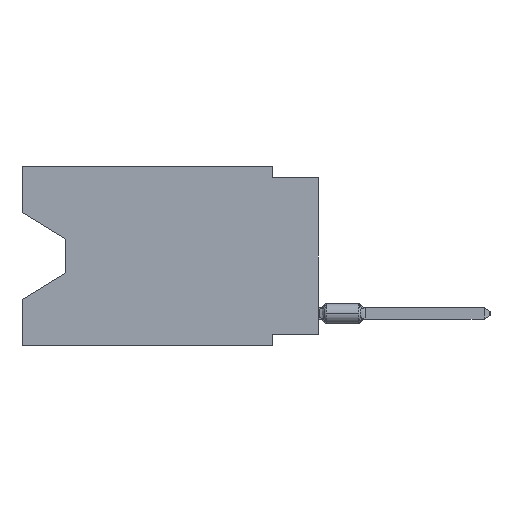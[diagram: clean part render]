
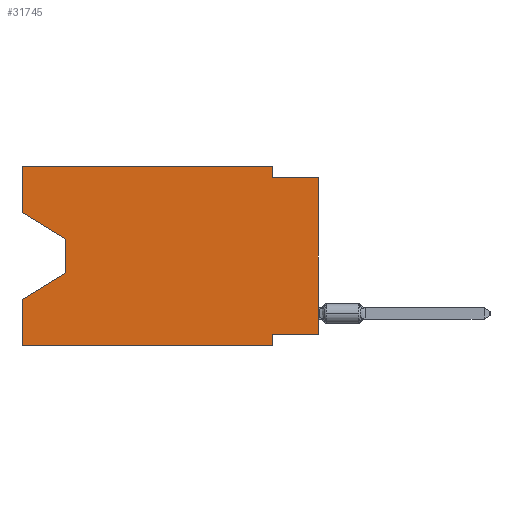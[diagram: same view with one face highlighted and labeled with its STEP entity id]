
A CAD part, left-side view. The second image highlights one B-rep face of the part: STEP entity #31745.
In plain terms, the highlighted planar face has unit normal (-1, 0, 0).
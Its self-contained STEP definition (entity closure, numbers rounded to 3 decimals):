
#317 = CARTESIAN_POINT ( 'NONE',  ( 0., 2.54, 0. ) ) ;
#794 = CARTESIAN_POINT ( 'NONE',  ( 0., 16.383, -7.36 ) ) ;
#2900 = EDGE_CURVE ( 'NONE', #40941, #24590, #13201, .T. ) ;
#3535 = CARTESIAN_POINT ( 'NONE',  ( 0., 2.54, -9.271 ) ) ;
#3606 = ORIENTED_EDGE ( 'NONE', *, *, #37681, .F. ) ;
#3652 = EDGE_CURVE ( 'NONE', #67904, #61742, #54714, .T. ) ;
#5133 = EDGE_CURVE ( 'NONE', #24590, #61742, #12142, .T. ) ;
#5158 = DIRECTION ( 'NONE',  ( 0., 0., -1. ) ) ;
#6600 = CARTESIAN_POINT ( 'NONE',  ( 0., 0., -0.635 ) ) ;
#6945 = ORIENTED_EDGE ( 'NONE', *, *, #54224, .T. ) ;
#7548 = EDGE_LOOP ( 'NONE', ( #6945, #16063, #22854, #64607, #65771, #75568, #11442, #66513, #3606, #39888, #7918, #61162 ) ) ;
#7918 = ORIENTED_EDGE ( 'NONE', *, *, #39443, .F. ) ;
#9223 = VECTOR ( 'NONE', #51706, 1000. ) ;
#10031 = EDGE_CURVE ( 'NONE', #40941, #60009, #31237, .T. ) ;
#11442 = ORIENTED_EDGE ( 'NONE', *, *, #2900, .F. ) ;
#12142 = LINE ( 'NONE', #12539, #59443 ) ;
#12539 = CARTESIAN_POINT ( 'NONE',  ( 0., 2.54, -9.906 ) ) ;
#12834 = EDGE_CURVE ( 'NONE', #67904, #27553, #40180, .T. ) ;
#13201 = LINE ( 'NONE', #73560, #40189 ) ;
#13399 = CARTESIAN_POINT ( 'NONE',  ( 0., 16.383, -9.906 ) ) ;
#16031 = VERTEX_POINT ( 'NONE', #59079 ) ;
#16063 = ORIENTED_EDGE ( 'NONE', *, *, #67375, .T. ) ;
#18263 = FACE_OUTER_BOUND ( 'NONE', #7548, .T. ) ;
#19189 = LINE ( 'NONE', #44994, #19703 ) ;
#19703 = VECTOR ( 'NONE', #19977, 1000. ) ;
#19977 = DIRECTION ( 'NONE',  ( 0., 0., -1. ) ) ;
#22854 = ORIENTED_EDGE ( 'NONE', *, *, #23159, .T. ) ;
#23034 = CARTESIAN_POINT ( 'NONE',  ( 0., 13.97, -5.893 ) ) ;
#23159 = EDGE_CURVE ( 'NONE', #16031, #27553, #48436, .T. ) ;
#24590 = VERTEX_POINT ( 'NONE', #3535 ) ;
#24606 = DIRECTION ( 'NONE',  ( 1., 0., 0. ) ) ;
#25218 = DIRECTION ( 'NONE',  ( 0., 0., -1. ) ) ;
#25721 = VERTEX_POINT ( 'NONE', #63692 ) ;
#27425 = CARTESIAN_POINT ( 'NONE',  ( 0., 0., -9.271 ) ) ;
#27553 = VERTEX_POINT ( 'NONE', #794 ) ;
#28257 = DIRECTION ( 'NONE',  ( 0., 0., 1. ) ) ;
#29636 = LINE ( 'NONE', #30027, #42923 ) ;
#30027 = CARTESIAN_POINT ( 'NONE',  ( 0., 16.383, -2.546 ) ) ;
#30146 = VECTOR ( 'NONE', #28257, 1000. ) ;
#30824 = DIRECTION ( 'NONE',  ( 0., -1., 0. ) ) ;
#31237 = LINE ( 'NONE', #37596, #67380 ) ;
#31328 = VECTOR ( 'NONE', #30824, 1000. ) ;
#31745 = ADVANCED_FACE ( 'NONE', ( #18263 ), #48042, .F. ) ;
#32896 = AXIS2_PLACEMENT_3D ( 'NONE', #42490, #24606, #5158 ) ;
#34213 = LINE ( 'NONE', #65194, #30146 ) ;
#37596 = CARTESIAN_POINT ( 'NONE',  ( 0., 0., 0. ) ) ;
#37681 = EDGE_CURVE ( 'NONE', #68597, #60009, #49102, .T. ) ;
#38248 = CARTESIAN_POINT ( 'NONE',  ( 0., 2.54, -0.635 ) ) ;
#38661 = CARTESIAN_POINT ( 'NONE',  ( 0., 16.383, 0. ) ) ;
#38982 = VECTOR ( 'NONE', #43185, 1000. ) ;
#39041 = LINE ( 'NONE', #38661, #71755 ) ;
#39443 = EDGE_CURVE ( 'NONE', #25721, #65677, #39041, .T. ) ;
#39522 = VERTEX_POINT ( 'NONE', #64465 ) ;
#39888 = ORIENTED_EDGE ( 'NONE', *, *, #53935, .F. ) ;
#40180 = LINE ( 'NONE', #64412, #9223 ) ;
#40189 = VECTOR ( 'NONE', #61636, 1000. ) ;
#40941 = VERTEX_POINT ( 'NONE', #27425 ) ;
#41727 = VECTOR ( 'NONE', #54413, 1000. ) ;
#42490 = CARTESIAN_POINT ( 'NONE',  ( 0., 16.383, 0. ) ) ;
#42826 = DIRECTION ( 'NONE',  ( 0., 0., -1. ) ) ;
#42923 = VECTOR ( 'NONE', #47514, 1000. ) ;
#43185 = DIRECTION ( 'NONE',  ( 0., -1., 0. ) ) ;
#43878 = CARTESIAN_POINT ( 'NONE',  ( 0., 16.383, -9.906 ) ) ;
#44994 = CARTESIAN_POINT ( 'NONE',  ( 0., 13.97, -4.013 ) ) ;
#47302 = CARTESIAN_POINT ( 'NONE',  ( 0., 2.54, -9.906 ) ) ;
#47514 = DIRECTION ( 'NONE',  ( 0., -0.855, -0.519 ) ) ;
#48042 = PLANE ( 'NONE',  #32896 ) ;
#48436 = LINE ( 'NONE', #23034, #41727 ) ;
#49102 = LINE ( 'NONE', #6600, #31328 ) ;
#51706 = DIRECTION ( 'NONE',  ( 0., 0., 1. ) ) ;
#53387 = EDGE_CURVE ( 'NONE', #39522, #25721, #34213, .T. ) ;
#53935 = EDGE_CURVE ( 'NONE', #65677, #68597, #54742, .T. ) ;
#54224 = EDGE_CURVE ( 'NONE', #39522, #59532, #29636, .T. ) ;
#54413 = DIRECTION ( 'NONE',  ( 0., 0.855, -0.519 ) ) ;
#54714 = LINE ( 'NONE', #13399, #38982 ) ;
#54742 = LINE ( 'NONE', #317, #74623 ) ;
#59079 = CARTESIAN_POINT ( 'NONE',  ( 0., 13.97, -5.893 ) ) ;
#59443 = VECTOR ( 'NONE', #25218, 1000. ) ;
#59532 = VERTEX_POINT ( 'NONE', #74659 ) ;
#59787 = CARTESIAN_POINT ( 'NONE',  ( 0., 0., -0.635 ) ) ;
#59808 = CARTESIAN_POINT ( 'NONE',  ( 0., 2.54, 0. ) ) ;
#60009 = VERTEX_POINT ( 'NONE', #59787 ) ;
#60640 = DIRECTION ( 'NONE',  ( 0., 0., 1. ) ) ;
#61162 = ORIENTED_EDGE ( 'NONE', *, *, #53387, .F. ) ;
#61636 = DIRECTION ( 'NONE',  ( 0., 1., 0. ) ) ;
#61742 = VERTEX_POINT ( 'NONE', #47302 ) ;
#63683 = DIRECTION ( 'NONE',  ( 0., -1., 0. ) ) ;
#63692 = CARTESIAN_POINT ( 'NONE',  ( 0., 16.383, 0. ) ) ;
#64412 = CARTESIAN_POINT ( 'NONE',  ( 0., 16.383, 0. ) ) ;
#64465 = CARTESIAN_POINT ( 'NONE',  ( 0., 16.383, -2.546 ) ) ;
#64607 = ORIENTED_EDGE ( 'NONE', *, *, #12834, .F. ) ;
#65194 = CARTESIAN_POINT ( 'NONE',  ( 0., 16.383, 0. ) ) ;
#65677 = VERTEX_POINT ( 'NONE', #59808 ) ;
#65771 = ORIENTED_EDGE ( 'NONE', *, *, #3652, .T. ) ;
#66513 = ORIENTED_EDGE ( 'NONE', *, *, #10031, .T. ) ;
#67375 = EDGE_CURVE ( 'NONE', #59532, #16031, #19189, .T. ) ;
#67380 = VECTOR ( 'NONE', #60640, 1000. ) ;
#67904 = VERTEX_POINT ( 'NONE', #43878 ) ;
#68597 = VERTEX_POINT ( 'NONE', #38248 ) ;
#71755 = VECTOR ( 'NONE', #63683, 1000. ) ;
#73560 = CARTESIAN_POINT ( 'NONE',  ( 0., 0., -9.271 ) ) ;
#74623 = VECTOR ( 'NONE', #42826, 1000. ) ;
#74659 = CARTESIAN_POINT ( 'NONE',  ( 0., 13.97, -4.013 ) ) ;
#75568 = ORIENTED_EDGE ( 'NONE', *, *, #5133, .F. ) ;
